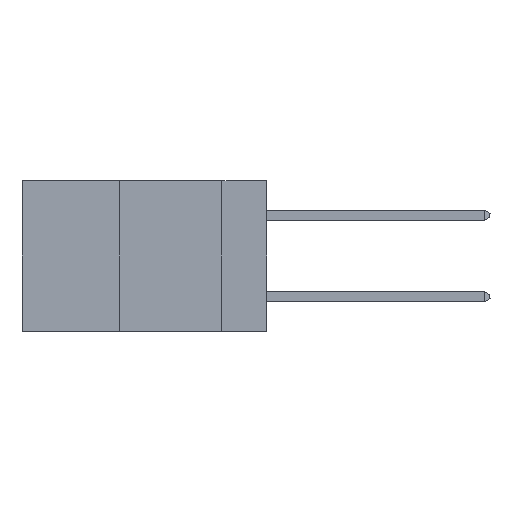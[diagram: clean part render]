
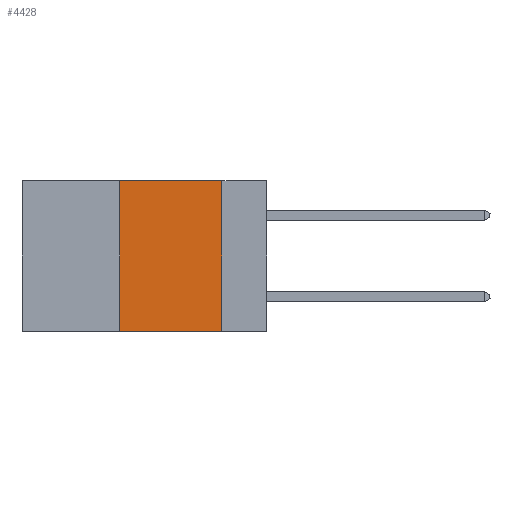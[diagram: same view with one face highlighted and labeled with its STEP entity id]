
A CAD part, left-side view. The second image highlights one B-rep face of the part: STEP entity #4428.
In plain terms, the highlighted planar face has unit normal (-1, 0, 0).
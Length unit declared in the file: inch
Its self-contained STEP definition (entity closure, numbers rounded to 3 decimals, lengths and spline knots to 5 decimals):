
#603 = VERTEX_POINT ( 'NONE', #17387 ) ;
#1854 = LINE ( 'NONE', #39447, #3963 ) ;
#2664 = FACE_OUTER_BOUND ( 'NONE', #28695, .T. ) ;
#3963 = VECTOR ( 'NONE', #19025, 39.37008 ) ;
#4428 = ADVANCED_FACE ( 'NONE', ( #2664 ), #35246, .F. ) ;
#5915 = VECTOR ( 'NONE', #12230, 39.37008 ) ;
#6018 = DIRECTION ( 'NONE',  ( 0., 0., 1. ) ) ;
#6072 = DIRECTION ( 'NONE',  ( 0., 0., -1. ) ) ;
#6222 = CARTESIAN_POINT ( 'NONE',  ( 0., 0.11, 0. ) ) ;
#6667 = EDGE_CURVE ( 'NONE', #24709, #19884, #10994, .T. ) ;
#7116 = DIRECTION ( 'NONE',  ( 0., 0., -1. ) ) ;
#7685 = ORIENTED_EDGE ( 'NONE', *, *, #12665, .F. ) ;
#9139 = ORIENTED_EDGE ( 'NONE', *, *, #36050, .T. ) ;
#10994 = LINE ( 'NONE', #17264, #26309 ) ;
#12230 = DIRECTION ( 'NONE',  ( 0., -1., 0. ) ) ;
#12665 = EDGE_CURVE ( 'NONE', #39996, #24709, #1854, .T. ) ;
#13295 = ORIENTED_EDGE ( 'NONE', *, *, #6667, .F. ) ;
#14764 = CARTESIAN_POINT ( 'NONE',  ( 0., 0.36, 0. ) ) ;
#16230 = CARTESIAN_POINT ( 'NONE',  ( 0., 0.6, 0. ) ) ;
#17264 = CARTESIAN_POINT ( 'NONE',  ( 0., 0.11, 0. ) ) ;
#17387 = CARTESIAN_POINT ( 'NONE',  ( 0., 0.36, -0.37 ) ) ;
#19025 = DIRECTION ( 'NONE',  ( 0., -1., 0. ) ) ;
#19111 = CARTESIAN_POINT ( 'NONE',  ( 0., 0.6, -0.37 ) ) ;
#19273 = CARTESIAN_POINT ( 'NONE',  ( 0., 0.11, -0.37 ) ) ;
#19403 = CARTESIAN_POINT ( 'NONE',  ( 0., 0.36, 0. ) ) ;
#19884 = VERTEX_POINT ( 'NONE', #19273 ) ;
#20413 = LINE ( 'NONE', #14764, #43010 ) ;
#24709 = VERTEX_POINT ( 'NONE', #6222 ) ;
#25457 = DIRECTION ( 'NONE',  ( 1., 0., 0. ) ) ;
#26309 = VECTOR ( 'NONE', #7116, 39.37008 ) ;
#26951 = EDGE_CURVE ( 'NONE', #603, #39996, #20413, .T. ) ;
#28695 = EDGE_LOOP ( 'NONE', ( #13295, #7685, #29814, #9139 ) ) ;
#29814 = ORIENTED_EDGE ( 'NONE', *, *, #26951, .F. ) ;
#32759 = LINE ( 'NONE', #19111, #5915 ) ;
#35246 = PLANE ( 'NONE',  #36066 ) ;
#36050 = EDGE_CURVE ( 'NONE', #603, #19884, #32759, .T. ) ;
#36066 = AXIS2_PLACEMENT_3D ( 'NONE', #16230, #25457, #6072 ) ;
#39447 = CARTESIAN_POINT ( 'NONE',  ( 0., 0.6, 0. ) ) ;
#39996 = VERTEX_POINT ( 'NONE', #19403 ) ;
#43010 = VECTOR ( 'NONE', #6018, 39.37008 ) ;
